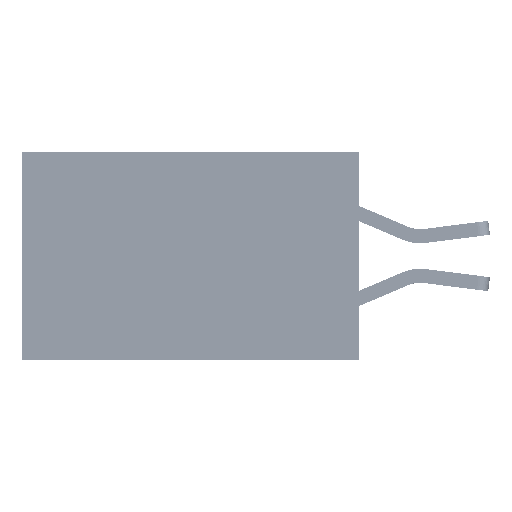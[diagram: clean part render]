
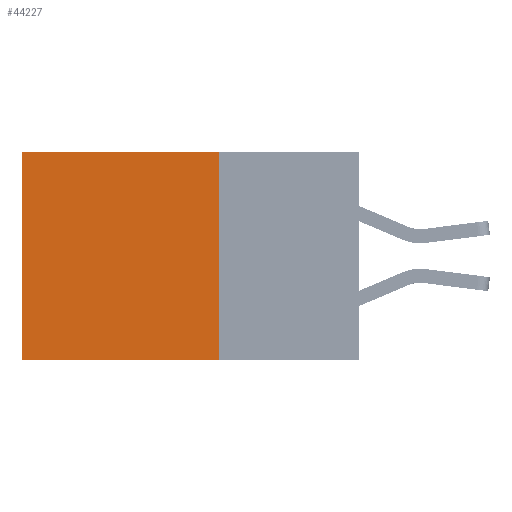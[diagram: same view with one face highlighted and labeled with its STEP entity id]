
A CAD part, left-side view. The second image highlights one B-rep face of the part: STEP entity #44227.
In plain terms, the highlighted planar face has unit normal (-1, 0, 0).
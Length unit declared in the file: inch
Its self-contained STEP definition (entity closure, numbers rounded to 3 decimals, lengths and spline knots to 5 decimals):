
#1285 = VERTEX_POINT ( 'NONE', #47439 ) ;
#1466 = LINE ( 'NONE', #40409, #37840 ) ;
#1473 = EDGE_CURVE ( 'NONE', #1285, #2009, #1466, .T. ) ;
#2009 = VERTEX_POINT ( 'NONE', #15895 ) ;
#4866 = DIRECTION ( 'NONE',  ( 0., 1., 0. ) ) ;
#6594 = DIRECTION ( 'NONE',  ( 0., 0., -1. ) ) ;
#10071 = PLANE ( 'NONE',  #47778 ) ;
#11227 = LINE ( 'NONE', #23181, #43856 ) ;
#14935 = LINE ( 'NONE', #19597, #25504 ) ;
#15572 = CARTESIAN_POINT ( 'NONE',  ( 0.2875, 0.6, 0. ) ) ;
#15895 = CARTESIAN_POINT ( 'NONE',  ( 0.2875, 0.6, 0. ) ) ;
#18637 = DIRECTION ( 'NONE',  ( 1., 0., 0. ) ) ;
#19597 = CARTESIAN_POINT ( 'NONE',  ( 0.2875, 0.25, -0.37 ) ) ;
#23181 = CARTESIAN_POINT ( 'NONE',  ( 0.2875, 0.25, 0. ) ) ;
#23770 = CARTESIAN_POINT ( 'NONE',  ( 0.2875, 0.25, -0.37 ) ) ;
#25434 = ORIENTED_EDGE ( 'NONE', *, *, #31177, .F. ) ;
#25504 = VECTOR ( 'NONE', #35416, 39.37008 ) ;
#27127 = EDGE_CURVE ( 'NONE', #2009, #50415, #43591, .T. ) ;
#31177 = EDGE_CURVE ( 'NONE', #1285, #49057, #11227, .T. ) ;
#33159 = VECTOR ( 'NONE', #51121, 39.37008 ) ;
#33932 = FACE_OUTER_BOUND ( 'NONE', #48635, .T. ) ;
#35416 = DIRECTION ( 'NONE',  ( 0., 1., 0. ) ) ;
#36498 = EDGE_CURVE ( 'NONE', #49057, #50415, #14935, .T. ) ;
#37314 = DIRECTION ( 'NONE',  ( 0., 0., -1. ) ) ;
#37840 = VECTOR ( 'NONE', #4866, 39.37008 ) ;
#38970 = ORIENTED_EDGE ( 'NONE', *, *, #1473, .T. ) ;
#40409 = CARTESIAN_POINT ( 'NONE',  ( 0.2875, 0.25, 0. ) ) ;
#41737 = ORIENTED_EDGE ( 'NONE', *, *, #36498, .F. ) ;
#43591 = LINE ( 'NONE', #15572, #33159 ) ;
#43856 = VECTOR ( 'NONE', #6594, 39.37008 ) ;
#44227 = ADVANCED_FACE ( 'NONE', ( #33932 ), #10071, .F. ) ;
#46131 = CARTESIAN_POINT ( 'NONE',  ( 0.2875, 0.25, 0. ) ) ;
#47113 = ORIENTED_EDGE ( 'NONE', *, *, #27127, .T. ) ;
#47439 = CARTESIAN_POINT ( 'NONE',  ( 0.2875, 0.25, 0. ) ) ;
#47778 = AXIS2_PLACEMENT_3D ( 'NONE', #46131, #18637, #37314 ) ;
#48635 = EDGE_LOOP ( 'NONE', ( #47113, #41737, #25434, #38970 ) ) ;
#49057 = VERTEX_POINT ( 'NONE', #23770 ) ;
#50415 = VERTEX_POINT ( 'NONE', #50580 ) ;
#50580 = CARTESIAN_POINT ( 'NONE',  ( 0.2875, 0.6, -0.37 ) ) ;
#51121 = DIRECTION ( 'NONE',  ( 0., 0., -1. ) ) ;
